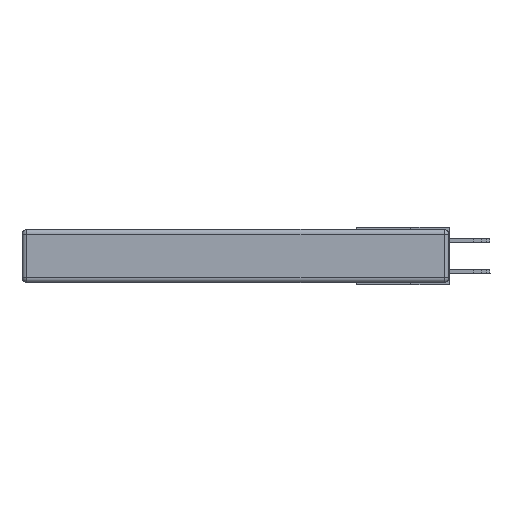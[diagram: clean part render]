
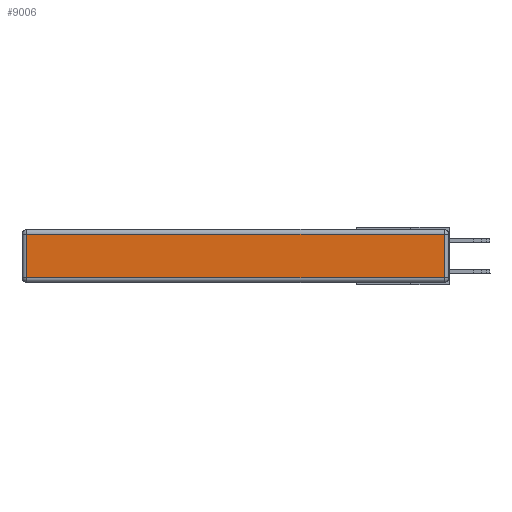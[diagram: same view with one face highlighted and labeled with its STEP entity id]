
A CAD part, left-side view. The second image highlights one B-rep face of the part: STEP entity #9006.
In plain terms, the highlighted planar face has unit normal (-1, 0, 0).
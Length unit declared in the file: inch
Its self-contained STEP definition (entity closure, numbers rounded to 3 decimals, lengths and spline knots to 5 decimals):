
#1857 = DIRECTION ( 'NONE',  ( -1., 0., 0. ) ) ;
#2430 = VECTOR ( 'NONE', #5128, 39.37008 ) ;
#2597 = EDGE_LOOP ( 'NONE', ( #22373, #20260, #6181, #9425 ) ) ;
#2614 = CARTESIAN_POINT ( 'NONE',  ( 0., 0.03, -0.313 ) ) ;
#2934 = VECTOR ( 'NONE', #22616, 39.37008 ) ;
#5128 = DIRECTION ( 'NONE',  ( 0., 0., 1. ) ) ;
#5730 = CARTESIAN_POINT ( 'NONE',  ( 0., 2.72, -0.343 ) ) ;
#6181 = ORIENTED_EDGE ( 'NONE', *, *, #16671, .T. ) ;
#7062 = AXIS2_PLACEMENT_3D ( 'NONE', #13387, #1857, #23079 ) ;
#7429 = VERTEX_POINT ( 'NONE', #8632 ) ;
#7724 = VERTEX_POINT ( 'NONE', #9527 ) ;
#8592 = LINE ( 'NONE', #22113, #13708 ) ;
#8632 = CARTESIAN_POINT ( 'NONE',  ( 0., 2.72, -0.03 ) ) ;
#8903 = VECTOR ( 'NONE', #11813, 39.37008 ) ;
#9006 = ADVANCED_FACE ( 'NONE', ( #17428 ), #11438, .T. ) ;
#9075 = EDGE_CURVE ( 'NONE', #7429, #18976, #15316, .T. ) ;
#9208 = VERTEX_POINT ( 'NONE', #2614 ) ;
#9425 = ORIENTED_EDGE ( 'NONE', *, *, #9075, .T. ) ;
#9527 = CARTESIAN_POINT ( 'NONE',  ( 0., 0.03, -0.03 ) ) ;
#10552 = DIRECTION ( 'NONE',  ( 0., 1., 0. ) ) ;
#10583 = EDGE_CURVE ( 'NONE', #18976, #9208, #14321, .T. ) ;
#11438 = PLANE ( 'NONE',  #7062 ) ;
#11813 = DIRECTION ( 'NONE',  ( 0., -1., 0. ) ) ;
#12503 = CARTESIAN_POINT ( 'NONE',  ( 0., 0.03, -0.343 ) ) ;
#13387 = CARTESIAN_POINT ( 'NONE',  ( 0., 0., -0.343 ) ) ;
#13708 = VECTOR ( 'NONE', #10552, 39.37008 ) ;
#14321 = LINE ( 'NONE', #23358, #8903 ) ;
#15316 = LINE ( 'NONE', #5730, #2934 ) ;
#16671 = EDGE_CURVE ( 'NONE', #7724, #7429, #8592, .T. ) ;
#17428 = FACE_OUTER_BOUND ( 'NONE', #2597, .T. ) ;
#17787 = LINE ( 'NONE', #12503, #2430 ) ;
#18828 = EDGE_CURVE ( 'NONE', #9208, #7724, #17787, .T. ) ;
#18976 = VERTEX_POINT ( 'NONE', #20280 ) ;
#20260 = ORIENTED_EDGE ( 'NONE', *, *, #18828, .T. ) ;
#20280 = CARTESIAN_POINT ( 'NONE',  ( 0., 2.72, -0.313 ) ) ;
#22113 = CARTESIAN_POINT ( 'NONE',  ( 0., 2.75, -0.03 ) ) ;
#22373 = ORIENTED_EDGE ( 'NONE', *, *, #10583, .T. ) ;
#22616 = DIRECTION ( 'NONE',  ( 0., 0., -1. ) ) ;
#23079 = DIRECTION ( 'NONE',  ( 0., 0., 1. ) ) ;
#23358 = CARTESIAN_POINT ( 'NONE',  ( 0., 0., -0.313 ) ) ;
